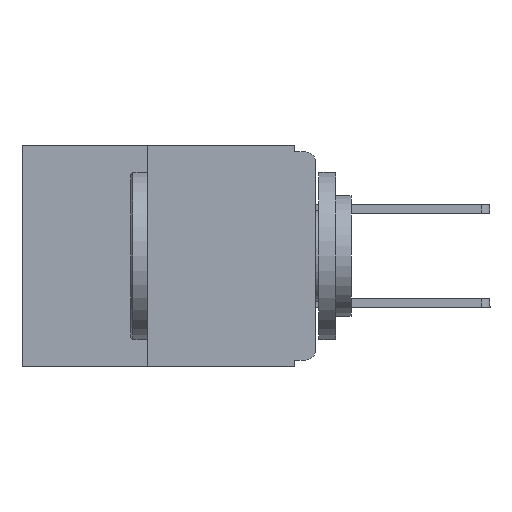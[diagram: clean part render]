
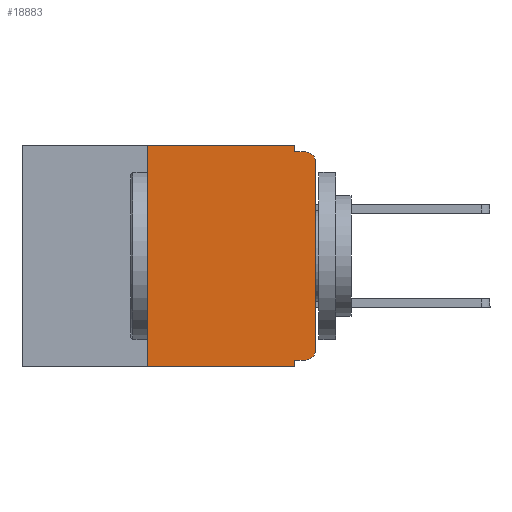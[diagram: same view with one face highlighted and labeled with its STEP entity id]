
A CAD part, left-side view. The second image highlights one B-rep face of the part: STEP entity #18883.
In plain terms, the highlighted planar face has unit normal (-1, 0, 0).
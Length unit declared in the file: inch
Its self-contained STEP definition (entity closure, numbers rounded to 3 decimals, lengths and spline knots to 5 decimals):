
#206 = ORIENTED_EDGE ( 'NONE', *, *, #21473, .F. ) ;
#573 = VERTEX_POINT ( 'NONE', #13996 ) ;
#923 = EDGE_CURVE ( 'NONE', #6005, #10028, #27970, .T. ) ;
#1049 = CARTESIAN_POINT ( 'NONE',  ( 0., 0.25, 0. ) ) ;
#1466 = DIRECTION ( 'NONE',  ( 0., 0., 1. ) ) ;
#1551 = DIRECTION ( 'NONE',  ( -1., 0., 0. ) ) ;
#1749 = CIRCLE ( 'NONE', #25803, 0.015 ) ;
#1796 = ORIENTED_EDGE ( 'NONE', *, *, #2403, .F. ) ;
#2026 = LINE ( 'NONE', #4192, #19521 ) ;
#2403 = EDGE_CURVE ( 'NONE', #14759, #7332, #10701, .T. ) ;
#2722 = LINE ( 'NONE', #12950, #14251 ) ;
#2920 = EDGE_CURVE ( 'NONE', #25941, #10028, #3892, .T. ) ;
#3814 = LINE ( 'NONE', #24274, #27779 ) ;
#3892 = LINE ( 'NONE', #7337, #27156 ) ;
#4115 = VECTOR ( 'NONE', #14811, 39.37008 ) ;
#4192 = CARTESIAN_POINT ( 'NONE',  ( 0., 0., -0.01 ) ) ;
#4467 = DIRECTION ( 'NONE',  ( 0., -1., 0. ) ) ;
#4606 = CARTESIAN_POINT ( 'NONE',  ( 0., 0.031, -0.33 ) ) ;
#4911 = EDGE_CURVE ( 'NONE', #18185, #6005, #22161, .T. ) ;
#5575 = ORIENTED_EDGE ( 'NONE', *, *, #22456, .F. ) ;
#6005 = VERTEX_POINT ( 'NONE', #7209 ) ;
#7096 = DIRECTION ( 'NONE',  ( 0., 0., 1. ) ) ;
#7148 = CARTESIAN_POINT ( 'NONE',  ( 0., 0.015, -0.025 ) ) ;
#7209 = CARTESIAN_POINT ( 'NONE',  ( 0., 0.031, -0.32 ) ) ;
#7327 = CARTESIAN_POINT ( 'NONE',  ( 0., 0.015, -0.32 ) ) ;
#7332 = VERTEX_POINT ( 'NONE', #24325 ) ;
#7337 = CARTESIAN_POINT ( 'NONE',  ( 0., 0.437, -0.33 ) ) ;
#7843 = CARTESIAN_POINT ( 'NONE',  ( 0., 0., -0.32 ) ) ;
#8102 = EDGE_CURVE ( 'NONE', #23744, #16065, #18236, .T. ) ;
#8653 = DIRECTION ( 'NONE',  ( 0., -1., 0. ) ) ;
#8731 = CARTESIAN_POINT ( 'NONE',  ( 0., 0.015, -0.01 ) ) ;
#9447 = DIRECTION ( 'NONE',  ( 0., 0., -1. ) ) ;
#10028 = VERTEX_POINT ( 'NONE', #11418 ) ;
#10281 = ORIENTED_EDGE ( 'NONE', *, *, #23365, .F. ) ;
#10701 = LINE ( 'NONE', #19912, #27876 ) ;
#10822 = DIRECTION ( 'NONE',  ( 0., 0., -1. ) ) ;
#10932 = VECTOR ( 'NONE', #7096, 39.37008 ) ;
#11182 = ORIENTED_EDGE ( 'NONE', *, *, #923, .F. ) ;
#11418 = CARTESIAN_POINT ( 'NONE',  ( 0., 0.031, -0.33 ) ) ;
#12950 = CARTESIAN_POINT ( 'NONE',  ( 0., 0., 0. ) ) ;
#13732 = FACE_OUTER_BOUND ( 'NONE', #26442, .T. ) ;
#13934 = CARTESIAN_POINT ( 'NONE',  ( 0., 0.25, -0.33 ) ) ;
#13996 = CARTESIAN_POINT ( 'NONE',  ( 0., 0.031, -0.01 ) ) ;
#14232 = EDGE_CURVE ( 'NONE', #19007, #23744, #2722, .T. ) ;
#14251 = VECTOR ( 'NONE', #1466, 39.37008 ) ;
#14256 = AXIS2_PLACEMENT_3D ( 'NONE', #19119, #28019, #14751 ) ;
#14751 = DIRECTION ( 'NONE',  ( 0., 0., -1. ) ) ;
#14759 = VERTEX_POINT ( 'NONE', #1049 ) ;
#14811 = DIRECTION ( 'NONE',  ( 0., 1., 0. ) ) ;
#14905 = ORIENTED_EDGE ( 'NONE', *, *, #2920, .T. ) ;
#15339 = CARTESIAN_POINT ( 'NONE',  ( 0., 0.015, -0.305 ) ) ;
#15620 = CARTESIAN_POINT ( 'NONE',  ( 0., 0., -0.305 ) ) ;
#16023 = DIRECTION ( 'NONE',  ( 0., -1., 0. ) ) ;
#16054 = CARTESIAN_POINT ( 'NONE',  ( 0., 0.25, -0.33 ) ) ;
#16065 = VERTEX_POINT ( 'NONE', #8731 ) ;
#17563 = DIRECTION ( 'NONE',  ( 0., 0., -1. ) ) ;
#18185 = VERTEX_POINT ( 'NONE', #7327 ) ;
#18236 = CIRCLE ( 'NONE', #26860, 0.015 ) ;
#18411 = EDGE_CURVE ( 'NONE', #18185, #19007, #1749, .T. ) ;
#18883 = ADVANCED_FACE ( 'NONE', ( #13732 ), #23565, .F. ) ;
#19007 = VERTEX_POINT ( 'NONE', #15620 ) ;
#19119 = CARTESIAN_POINT ( 'NONE',  ( 0., 0.437, 0. ) ) ;
#19521 = VECTOR ( 'NONE', #8653, 39.37008 ) ;
#19912 = CARTESIAN_POINT ( 'NONE',  ( 0., 0.437, 0. ) ) ;
#21473 = EDGE_CURVE ( 'NONE', #573, #16065, #2026, .T. ) ;
#22161 = LINE ( 'NONE', #7843, #4115 ) ;
#22209 = LINE ( 'NONE', #13934, #10932 ) ;
#22456 = EDGE_CURVE ( 'NONE', #7332, #573, #3814, .T. ) ;
#22949 = DIRECTION ( 'NONE',  ( -1., 0., 0. ) ) ;
#23365 = EDGE_CURVE ( 'NONE', #25941, #14759, #22209, .T. ) ;
#23565 = PLANE ( 'NONE',  #14256 ) ;
#23744 = VERTEX_POINT ( 'NONE', #26444 ) ;
#24274 = CARTESIAN_POINT ( 'NONE',  ( 0., 0.031, 0. ) ) ;
#24325 = CARTESIAN_POINT ( 'NONE',  ( 0., 0.031, 0. ) ) ;
#24443 = ORIENTED_EDGE ( 'NONE', *, *, #14232, .T. ) ;
#25065 = ORIENTED_EDGE ( 'NONE', *, *, #4911, .F. ) ;
#25803 = AXIS2_PLACEMENT_3D ( 'NONE', #15339, #1551, #17563 ) ;
#25941 = VERTEX_POINT ( 'NONE', #16054 ) ;
#26442 = EDGE_LOOP ( 'NONE', ( #24443, #28520, #206, #5575, #1796, #10281, #14905, #11182, #25065, #27891 ) ) ;
#26444 = CARTESIAN_POINT ( 'NONE',  ( 0., 0., -0.025 ) ) ;
#26860 = AXIS2_PLACEMENT_3D ( 'NONE', #7148, #22949, #9447 ) ;
#27156 = VECTOR ( 'NONE', #4467, 39.37008 ) ;
#27293 = VECTOR ( 'NONE', #28554, 39.37008 ) ;
#27779 = VECTOR ( 'NONE', #10822, 39.37008 ) ;
#27876 = VECTOR ( 'NONE', #16023, 39.37008 ) ;
#27891 = ORIENTED_EDGE ( 'NONE', *, *, #18411, .T. ) ;
#27970 = LINE ( 'NONE', #4606, #27293 ) ;
#28019 = DIRECTION ( 'NONE',  ( 1., 0., 0. ) ) ;
#28520 = ORIENTED_EDGE ( 'NONE', *, *, #8102, .T. ) ;
#28554 = DIRECTION ( 'NONE',  ( 0., 0., -1. ) ) ;
